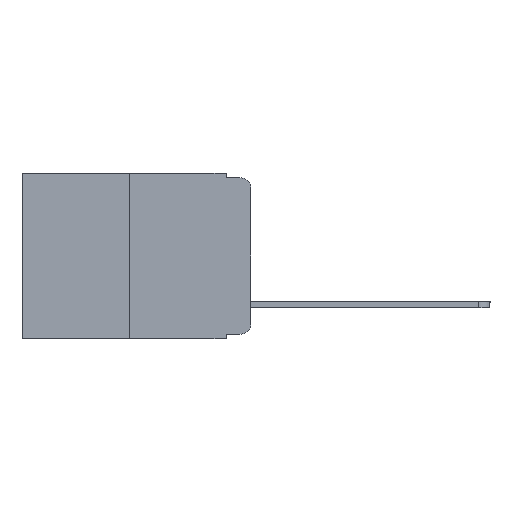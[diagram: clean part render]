
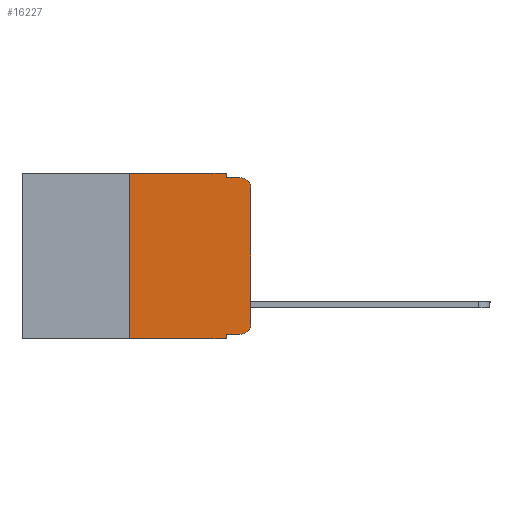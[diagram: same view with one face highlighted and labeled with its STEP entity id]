
A CAD part, left-side view. The second image highlights one B-rep face of the part: STEP entity #16227.
In plain terms, the highlighted planar face has unit normal (-1, 0, 0).
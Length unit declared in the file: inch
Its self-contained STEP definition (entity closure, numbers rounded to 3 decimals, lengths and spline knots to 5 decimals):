
#36 = VERTEX_POINT ( 'NONE', #17131 ) ;
#199 = LINE ( 'NONE', #13549, #8450 ) ;
#221 = EDGE_LOOP ( 'NONE', ( #8096, #15758, #2036, #15129, #16244, #9667, #12685, #10892, #3996, #2231 ) ) ;
#668 = VERTEX_POINT ( 'NONE', #16332 ) ;
#753 = DIRECTION ( 'NONE',  ( 0., -1., 0. ) ) ;
#1468 = DIRECTION ( 'NONE',  ( 0., -1., 0. ) ) ;
#2036 = ORIENTED_EDGE ( 'NONE', *, *, #8470, .F. ) ;
#2072 = LINE ( 'NONE', #10312, #4294 ) ;
#2231 = ORIENTED_EDGE ( 'NONE', *, *, #11081, .T. ) ;
#2300 = DIRECTION ( 'NONE',  ( -1., 0., 0. ) ) ;
#2330 = VECTOR ( 'NONE', #9113, 39.37008 ) ;
#2960 = AXIS2_PLACEMENT_3D ( 'NONE', #12801, #2300, #14119 ) ;
#3271 = LINE ( 'NONE', #12742, #3802 ) ;
#3458 = FACE_OUTER_BOUND ( 'NONE', #221, .T. ) ;
#3663 = DIRECTION ( 'NONE',  ( 0., 0., 1. ) ) ;
#3795 = CARTESIAN_POINT ( 'NONE',  ( 0., 0.25, 0. ) ) ;
#3802 = VECTOR ( 'NONE', #6172, 39.37008 ) ;
#3996 = ORIENTED_EDGE ( 'NONE', *, *, #6417, .T. ) ;
#4294 = VECTOR ( 'NONE', #753, 39.37008 ) ;
#4386 = DIRECTION ( 'NONE',  ( 0., 0., -1. ) ) ;
#4543 = CARTESIAN_POINT ( 'NONE',  ( 0., 0., -0.313 ) ) ;
#4614 = CARTESIAN_POINT ( 'NONE',  ( 0., 0.25, 0. ) ) ;
#4862 = DIRECTION ( 'NONE',  ( 0., 0., -1. ) ) ;
#4878 = VERTEX_POINT ( 'NONE', #4614 ) ;
#5190 = CARTESIAN_POINT ( 'NONE',  ( 0., 0.051, 0. ) ) ;
#5194 = CARTESIAN_POINT ( 'NONE',  ( 0., 0.051, -0.01 ) ) ;
#6165 = DIRECTION ( 'NONE',  ( 1., 0., 0. ) ) ;
#6172 = DIRECTION ( 'NONE',  ( 0., 0., -1. ) ) ;
#6389 = LINE ( 'NONE', #6660, #17297 ) ;
#6406 = DIRECTION ( 'NONE',  ( 0., -1., 0. ) ) ;
#6417 = EDGE_CURVE ( 'NONE', #16316, #14565, #199, .T. ) ;
#6660 = CARTESIAN_POINT ( 'NONE',  ( 0., 0.051, 0. ) ) ;
#7199 = EDGE_CURVE ( 'NONE', #11942, #4878, #13143, .T. ) ;
#7333 = LINE ( 'NONE', #14245, #15764 ) ;
#7481 = CARTESIAN_POINT ( 'NONE',  ( 0., 0.473, 0. ) ) ;
#7741 = CARTESIAN_POINT ( 'NONE',  ( 0., 0.02, -0.333 ) ) ;
#7891 = VECTOR ( 'NONE', #6406, 39.37008 ) ;
#8047 = VERTEX_POINT ( 'NONE', #4543 ) ;
#8096 = ORIENTED_EDGE ( 'NONE', *, *, #9168, .T. ) ;
#8331 = VERTEX_POINT ( 'NONE', #12644 ) ;
#8450 = VECTOR ( 'NONE', #1468, 39.37008 ) ;
#8470 = EDGE_CURVE ( 'NONE', #668, #8331, #15532, .T. ) ;
#8785 = PLANE ( 'NONE',  #15925 ) ;
#8953 = CIRCLE ( 'NONE', #14555, 0.02 ) ;
#9113 = DIRECTION ( 'NONE',  ( 0., 0., 1. ) ) ;
#9140 = CARTESIAN_POINT ( 'NONE',  ( 0., 0.25, -0.343 ) ) ;
#9168 = EDGE_CURVE ( 'NONE', #8047, #9421, #7333, .T. ) ;
#9200 = EDGE_CURVE ( 'NONE', #11942, #36, #2072, .T. ) ;
#9288 = CARTESIAN_POINT ( 'NONE',  ( 0., 0.473, 0. ) ) ;
#9421 = VERTEX_POINT ( 'NONE', #14954 ) ;
#9467 = VECTOR ( 'NONE', #17256, 39.37008 ) ;
#9667 = ORIENTED_EDGE ( 'NONE', *, *, #7199, .F. ) ;
#10312 = CARTESIAN_POINT ( 'NONE',  ( 0., 0.473, -0.343 ) ) ;
#10743 = EDGE_CURVE ( 'NONE', #16316, #36, #3271, .T. ) ;
#10892 = ORIENTED_EDGE ( 'NONE', *, *, #10743, .F. ) ;
#11041 = CARTESIAN_POINT ( 'NONE',  ( 0., 0.02, -0.03 ) ) ;
#11081 = EDGE_CURVE ( 'NONE', #14565, #8047, #14734, .T. ) ;
#11924 = LINE ( 'NONE', #9288, #9467 ) ;
#11942 = VERTEX_POINT ( 'NONE', #9140 ) ;
#12005 = DIRECTION ( 'NONE',  ( 0., 0., -1. ) ) ;
#12506 = VERTEX_POINT ( 'NONE', #5190 ) ;
#12644 = CARTESIAN_POINT ( 'NONE',  ( 0., 0.02, -0.01 ) ) ;
#12685 = ORIENTED_EDGE ( 'NONE', *, *, #9200, .T. ) ;
#12742 = CARTESIAN_POINT ( 'NONE',  ( 0., 0.051, 0. ) ) ;
#12801 = CARTESIAN_POINT ( 'NONE',  ( 0., 0.02, -0.313 ) ) ;
#13143 = LINE ( 'NONE', #3795, #2330 ) ;
#13549 = CARTESIAN_POINT ( 'NONE',  ( 0., 0.051, -0.333 ) ) ;
#13849 = EDGE_CURVE ( 'NONE', #12506, #668, #6389, .T. ) ;
#14119 = DIRECTION ( 'NONE',  ( 0., 0., -1. ) ) ;
#14245 = CARTESIAN_POINT ( 'NONE',  ( 0., 0., 0. ) ) ;
#14408 = CARTESIAN_POINT ( 'NONE',  ( 0., 0.051, -0.333 ) ) ;
#14555 = AXIS2_PLACEMENT_3D ( 'NONE', #11041, #16384, #4386 ) ;
#14565 = VERTEX_POINT ( 'NONE', #7741 ) ;
#14734 = CIRCLE ( 'NONE', #2960, 0.02 ) ;
#14954 = CARTESIAN_POINT ( 'NONE',  ( 0., 0., -0.03 ) ) ;
#15105 = EDGE_CURVE ( 'NONE', #4878, #12506, #11924, .T. ) ;
#15129 = ORIENTED_EDGE ( 'NONE', *, *, #13849, .F. ) ;
#15532 = LINE ( 'NONE', #5194, #7891 ) ;
#15758 = ORIENTED_EDGE ( 'NONE', *, *, #17003, .T. ) ;
#15764 = VECTOR ( 'NONE', #3663, 39.37008 ) ;
#15925 = AXIS2_PLACEMENT_3D ( 'NONE', #7481, #6165, #4862 ) ;
#16227 = ADVANCED_FACE ( 'NONE', ( #3458 ), #8785, .F. ) ;
#16244 = ORIENTED_EDGE ( 'NONE', *, *, #15105, .F. ) ;
#16316 = VERTEX_POINT ( 'NONE', #14408 ) ;
#16332 = CARTESIAN_POINT ( 'NONE',  ( 0., 0.051, -0.01 ) ) ;
#16384 = DIRECTION ( 'NONE',  ( -1., 0., 0. ) ) ;
#17003 = EDGE_CURVE ( 'NONE', #9421, #8331, #8953, .T. ) ;
#17131 = CARTESIAN_POINT ( 'NONE',  ( 0., 0.051, -0.343 ) ) ;
#17256 = DIRECTION ( 'NONE',  ( 0., -1., 0. ) ) ;
#17297 = VECTOR ( 'NONE', #12005, 39.37008 ) ;
